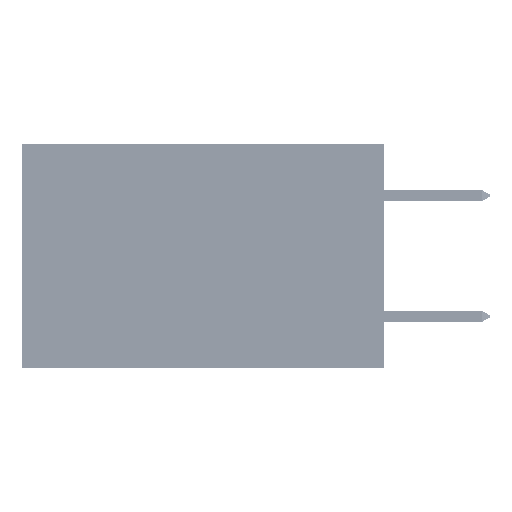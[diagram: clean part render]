
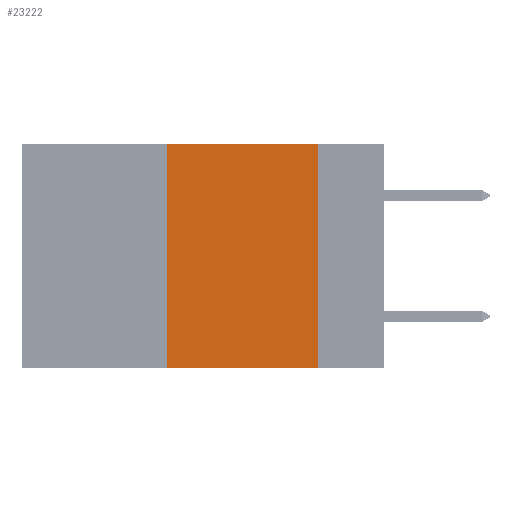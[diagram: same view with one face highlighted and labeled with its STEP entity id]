
A CAD part, left-side view. The second image highlights one B-rep face of the part: STEP entity #23222.
In plain terms, the highlighted planar face has unit normal (-1, 0, 0).
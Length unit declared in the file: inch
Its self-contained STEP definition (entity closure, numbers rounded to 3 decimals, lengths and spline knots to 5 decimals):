
#1274 = CARTESIAN_POINT ( 'NONE',  ( 0., 0.36, 0. ) ) ;
#1560 = AXIS2_PLACEMENT_3D ( 'NONE', #22689, #4777, #43598 ) ;
#1742 = VECTOR ( 'NONE', #42991, 39.37008 ) ;
#2532 = EDGE_LOOP ( 'NONE', ( #23265, #38182, #36504, #45710 ) ) ;
#4255 = LINE ( 'NONE', #31111, #20462 ) ;
#4306 = EDGE_CURVE ( 'NONE', #22171, #42741, #27753, .T. ) ;
#4777 = DIRECTION ( 'NONE',  ( 1., 0., 0. ) ) ;
#6530 = VECTOR ( 'NONE', #29983, 39.37008 ) ;
#6578 = EDGE_CURVE ( 'NONE', #22171, #26964, #9801, .T. ) ;
#7784 = CARTESIAN_POINT ( 'NONE',  ( 0., 0.6, 0. ) ) ;
#9390 = CARTESIAN_POINT ( 'NONE',  ( 0., 0.6, -0.37 ) ) ;
#9801 = LINE ( 'NONE', #19604, #24270 ) ;
#11294 = LINE ( 'NONE', #7784, #1742 ) ;
#18548 = CARTESIAN_POINT ( 'NONE',  ( 0., 0.11, -0.37 ) ) ;
#19604 = CARTESIAN_POINT ( 'NONE',  ( 0., 0.36, 0. ) ) ;
#20462 = VECTOR ( 'NONE', #41043, 39.37008 ) ;
#22171 = VERTEX_POINT ( 'NONE', #45517 ) ;
#22689 = CARTESIAN_POINT ( 'NONE',  ( 0., 0.6, 0. ) ) ;
#23222 = ADVANCED_FACE ( 'NONE', ( #43354 ), #26298, .F. ) ;
#23265 = ORIENTED_EDGE ( 'NONE', *, *, #31038, .F. ) ;
#24270 = VECTOR ( 'NONE', #40965, 39.37008 ) ;
#26298 = PLANE ( 'NONE',  #1560 ) ;
#26964 = VERTEX_POINT ( 'NONE', #1274 ) ;
#27753 = LINE ( 'NONE', #9390, #6530 ) ;
#29983 = DIRECTION ( 'NONE',  ( 0., -1., 0. ) ) ;
#31038 = EDGE_CURVE ( 'NONE', #36950, #42741, #4255, .T. ) ;
#31111 = CARTESIAN_POINT ( 'NONE',  ( 0., 0.11, 0. ) ) ;
#36504 = ORIENTED_EDGE ( 'NONE', *, *, #6578, .F. ) ;
#36950 = VERTEX_POINT ( 'NONE', #46039 ) ;
#38182 = ORIENTED_EDGE ( 'NONE', *, *, #41346, .F. ) ;
#40965 = DIRECTION ( 'NONE',  ( 0., 0., 1. ) ) ;
#41043 = DIRECTION ( 'NONE',  ( 0., 0., -1. ) ) ;
#41346 = EDGE_CURVE ( 'NONE', #26964, #36950, #11294, .T. ) ;
#42741 = VERTEX_POINT ( 'NONE', #18548 ) ;
#42991 = DIRECTION ( 'NONE',  ( 0., -1., 0. ) ) ;
#43354 = FACE_OUTER_BOUND ( 'NONE', #2532, .T. ) ;
#43598 = DIRECTION ( 'NONE',  ( 0., 0., -1. ) ) ;
#45517 = CARTESIAN_POINT ( 'NONE',  ( 0., 0.36, -0.37 ) ) ;
#45710 = ORIENTED_EDGE ( 'NONE', *, *, #4306, .T. ) ;
#46039 = CARTESIAN_POINT ( 'NONE',  ( 0., 0.11, 0. ) ) ;
